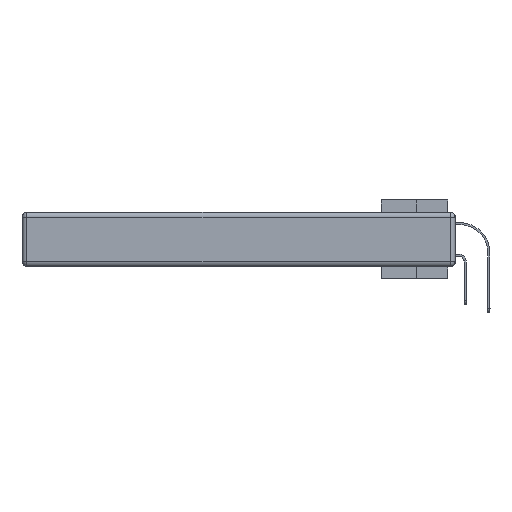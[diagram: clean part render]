
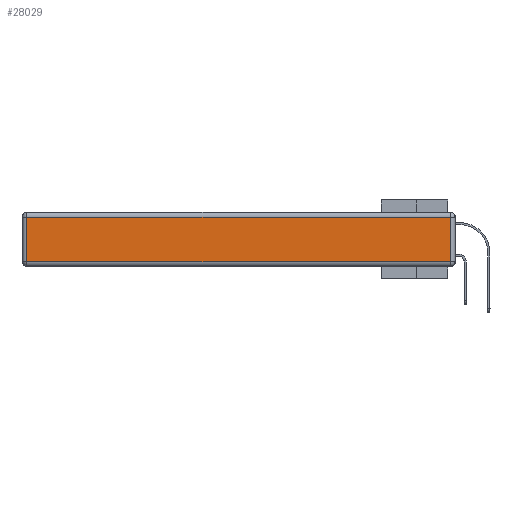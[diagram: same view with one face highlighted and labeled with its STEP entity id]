
A CAD part, left-side view. The second image highlights one B-rep face of the part: STEP entity #28029.
In plain terms, the highlighted planar face has unit normal (-1, 0, 0).
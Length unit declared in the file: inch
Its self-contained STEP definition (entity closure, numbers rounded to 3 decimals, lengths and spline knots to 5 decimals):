
#823 = VERTEX_POINT ( 'NONE', #29014 ) ;
#1348 = DIRECTION ( 'NONE',  ( 0., -1., 0. ) ) ;
#3211 = DIRECTION ( 'NONE',  ( 0., 1., 0. ) ) ;
#4446 = EDGE_CURVE ( 'NONE', #26276, #28853, #27080, .T. ) ;
#5567 = PLANE ( 'NONE',  #24439 ) ;
#5975 = CARTESIAN_POINT ( 'NONE',  ( 0., 0.03, -0.03 ) ) ;
#6035 = LINE ( 'NONE', #14267, #30122 ) ;
#6109 = CARTESIAN_POINT ( 'NONE',  ( 0., 0., -0.343 ) ) ;
#6308 = FACE_OUTER_BOUND ( 'NONE', #12118, .T. ) ;
#6627 = ORIENTED_EDGE ( 'NONE', *, *, #26854, .T. ) ;
#6855 = CARTESIAN_POINT ( 'NONE',  ( 0., 0.03, -0.343 ) ) ;
#8968 = EDGE_CURVE ( 'NONE', #36446, #823, #35214, .T. ) ;
#10150 = DIRECTION ( 'NONE',  ( 0., 0., -1. ) ) ;
#10343 = CARTESIAN_POINT ( 'NONE',  ( 0., 2.72, -0.343 ) ) ;
#12118 = EDGE_LOOP ( 'NONE', ( #6627, #34188, #22430, #33564 ) ) ;
#14267 = CARTESIAN_POINT ( 'NONE',  ( 0., 2.75, -0.03 ) ) ;
#14373 = CARTESIAN_POINT ( 'NONE',  ( 0., 0.03, -0.313 ) ) ;
#16989 = DIRECTION ( 'NONE',  ( 0., 0., 1. ) ) ;
#19114 = CARTESIAN_POINT ( 'NONE',  ( 0., 2.72, -0.03 ) ) ;
#20480 = VECTOR ( 'NONE', #10150, 39.37008 ) ;
#21784 = EDGE_CURVE ( 'NONE', #28853, #36446, #6035, .T. ) ;
#22430 = ORIENTED_EDGE ( 'NONE', *, *, #21784, .T. ) ;
#24439 = AXIS2_PLACEMENT_3D ( 'NONE', #6109, #31932, #16989 ) ;
#26276 = VERTEX_POINT ( 'NONE', #14373 ) ;
#26677 = VECTOR ( 'NONE', #35468, 39.37008 ) ;
#26832 = CARTESIAN_POINT ( 'NONE',  ( 0., 0., -0.313 ) ) ;
#26854 = EDGE_CURVE ( 'NONE', #823, #26276, #27021, .T. ) ;
#27021 = LINE ( 'NONE', #26832, #32088 ) ;
#27080 = LINE ( 'NONE', #6855, #26677 ) ;
#28029 = ADVANCED_FACE ( 'NONE', ( #6308 ), #5567, .T. ) ;
#28853 = VERTEX_POINT ( 'NONE', #5975 ) ;
#29014 = CARTESIAN_POINT ( 'NONE',  ( 0., 2.72, -0.313 ) ) ;
#30122 = VECTOR ( 'NONE', #3211, 39.37008 ) ;
#31932 = DIRECTION ( 'NONE',  ( -1., 0., 0. ) ) ;
#32088 = VECTOR ( 'NONE', #1348, 39.37008 ) ;
#33564 = ORIENTED_EDGE ( 'NONE', *, *, #8968, .T. ) ;
#34188 = ORIENTED_EDGE ( 'NONE', *, *, #4446, .T. ) ;
#35214 = LINE ( 'NONE', #10343, #20480 ) ;
#35468 = DIRECTION ( 'NONE',  ( 0., 0., 1. ) ) ;
#36446 = VERTEX_POINT ( 'NONE', #19114 ) ;
